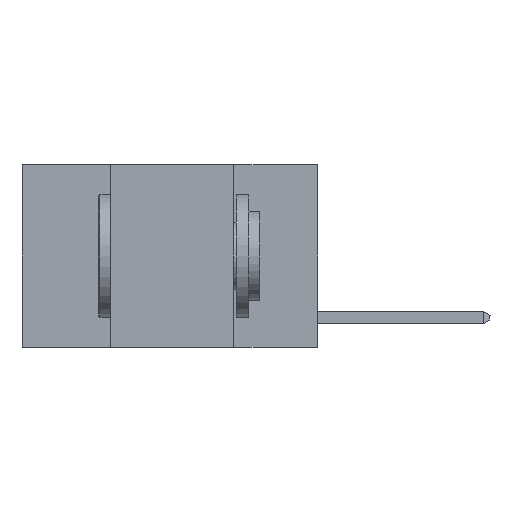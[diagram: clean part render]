
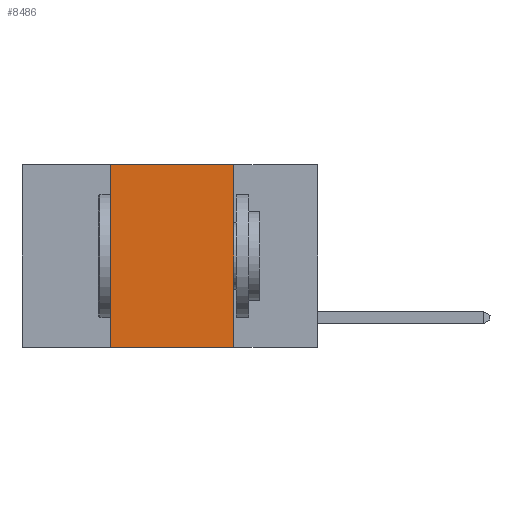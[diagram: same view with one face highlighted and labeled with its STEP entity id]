
A CAD part, left-side view. The second image highlights one B-rep face of the part: STEP entity #8486.
In plain terms, the highlighted planar face has unit normal (-1, 0, 0).
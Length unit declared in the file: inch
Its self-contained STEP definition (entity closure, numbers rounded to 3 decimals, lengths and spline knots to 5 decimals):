
#285 = EDGE_CURVE ( 'NONE', #5068, #8976, #9878, .T. ) ;
#725 = DIRECTION ( 'NONE',  ( 0., 0., -1. ) ) ;
#1156 = ORIENTED_EDGE ( 'NONE', *, *, #3100, .T. ) ;
#1625 = EDGE_CURVE ( 'NONE', #4642, #5068, #2770, .T. ) ;
#1860 = ORIENTED_EDGE ( 'NONE', *, *, #285, .F. ) ;
#1925 = CARTESIAN_POINT ( 'NONE',  ( 0., 0.17, 0. ) ) ;
#1937 = CARTESIAN_POINT ( 'NONE',  ( 0., 0.42, -0.37 ) ) ;
#1963 = VECTOR ( 'NONE', #3467, 39.37008 ) ;
#2019 = AXIS2_PLACEMENT_3D ( 'NONE', #3944, #7144, #725 ) ;
#2283 = VECTOR ( 'NONE', #9718, 39.37008 ) ;
#2583 = CARTESIAN_POINT ( 'NONE',  ( 0., 0.17, -0.37 ) ) ;
#2630 = CARTESIAN_POINT ( 'NONE',  ( 0., 0.17, 0. ) ) ;
#2717 = VECTOR ( 'NONE', #8404, 39.37008 ) ;
#2770 = LINE ( 'NONE', #7582, #2717 ) ;
#3100 = EDGE_CURVE ( 'NONE', #6460, #8976, #5509, .T. ) ;
#3177 = CARTESIAN_POINT ( 'NONE',  ( 0., 0.6, -0.37 ) ) ;
#3467 = DIRECTION ( 'NONE',  ( 0., 0., 1. ) ) ;
#3736 = VECTOR ( 'NONE', #7985, 39.37008 ) ;
#3944 = CARTESIAN_POINT ( 'NONE',  ( 0., 0.6, 0. ) ) ;
#4642 = VERTEX_POINT ( 'NONE', #7721 ) ;
#5068 = VERTEX_POINT ( 'NONE', #1925 ) ;
#5151 = CARTESIAN_POINT ( 'NONE',  ( 0., 0.42, 0. ) ) ;
#5160 = ORIENTED_EDGE ( 'NONE', *, *, #1625, .F. ) ;
#5495 = PLANE ( 'NONE',  #2019 ) ;
#5496 = EDGE_CURVE ( 'NONE', #6460, #4642, #7598, .T. ) ;
#5509 = LINE ( 'NONE', #3177, #3736 ) ;
#5928 = ORIENTED_EDGE ( 'NONE', *, *, #5496, .F. ) ;
#6460 = VERTEX_POINT ( 'NONE', #1937 ) ;
#7144 = DIRECTION ( 'NONE',  ( 1., 0., 0. ) ) ;
#7249 = FACE_OUTER_BOUND ( 'NONE', #9849, .T. ) ;
#7582 = CARTESIAN_POINT ( 'NONE',  ( 0., 0.6, 0. ) ) ;
#7598 = LINE ( 'NONE', #5151, #1963 ) ;
#7721 = CARTESIAN_POINT ( 'NONE',  ( 0., 0.42, 0. ) ) ;
#7985 = DIRECTION ( 'NONE',  ( 0., -1., 0. ) ) ;
#8404 = DIRECTION ( 'NONE',  ( 0., -1., 0. ) ) ;
#8486 = ADVANCED_FACE ( 'NONE', ( #7249 ), #5495, .F. ) ;
#8976 = VERTEX_POINT ( 'NONE', #2583 ) ;
#9718 = DIRECTION ( 'NONE',  ( 0., 0., -1. ) ) ;
#9849 = EDGE_LOOP ( 'NONE', ( #1860, #5160, #5928, #1156 ) ) ;
#9878 = LINE ( 'NONE', #2630, #2283 ) ;
